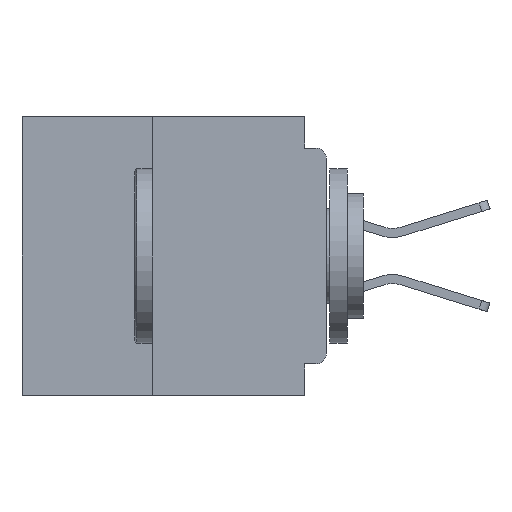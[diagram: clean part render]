
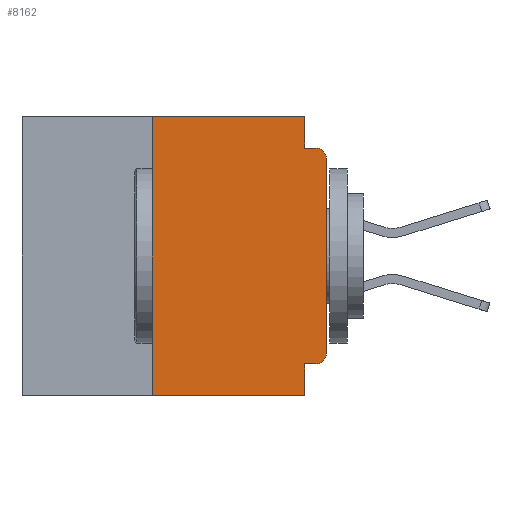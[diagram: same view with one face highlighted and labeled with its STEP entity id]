
A CAD part, left-side view. The second image highlights one B-rep face of the part: STEP entity #8162.
In plain terms, the highlighted planar face has unit normal (-1, 0, 0).
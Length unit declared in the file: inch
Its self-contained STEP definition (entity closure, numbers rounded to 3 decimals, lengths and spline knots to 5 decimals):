
#472 = DIRECTION ( 'NONE',  ( 0., 0., -1. ) ) ;
#591 = VECTOR ( 'NONE', #36430, 39.37008 ) ;
#720 = VECTOR ( 'NONE', #472, 39.37008 ) ;
#1626 = CARTESIAN_POINT ( 'NONE',  ( 0., 0., -0.045 ) ) ;
#1841 = VERTEX_POINT ( 'NONE', #35062 ) ;
#2257 = LINE ( 'NONE', #1626, #17665 ) ;
#2867 = VERTEX_POINT ( 'NONE', #30330 ) ;
#3822 = DIRECTION ( 'NONE',  ( 0., 0., -1. ) ) ;
#4302 = ORIENTED_EDGE ( 'NONE', *, *, #34693, .T. ) ;
#4424 = EDGE_CURVE ( 'NONE', #17316, #37207, #24760, .T. ) ;
#4809 = EDGE_LOOP ( 'NONE', ( #5668, #30930, #11366, #27231, #41354, #8035, #8741, #14211, #24919, #4302 ) ) ;
#5165 = AXIS2_PLACEMENT_3D ( 'NONE', #16802, #23419, #3822 ) ;
#5299 = CARTESIAN_POINT ( 'NONE',  ( 0., 0., -0.34 ) ) ;
#5668 = ORIENTED_EDGE ( 'NONE', *, *, #7527, .T. ) ;
#6003 = CARTESIAN_POINT ( 'NONE',  ( 0., 0.015, -0.045 ) ) ;
#6198 = CARTESIAN_POINT ( 'NONE',  ( 0., 0.437, -0.4 ) ) ;
#6359 = EDGE_CURVE ( 'NONE', #32791, #16453, #21707, .T. ) ;
#6423 = VECTOR ( 'NONE', #14970, 39.37008 ) ;
#7133 = CARTESIAN_POINT ( 'NONE',  ( 0., 0.031, -0.4 ) ) ;
#7527 = EDGE_CURVE ( 'NONE', #12212, #1841, #34368, .T. ) ;
#7808 = CIRCLE ( 'NONE', #42087, 0.015 ) ;
#8035 = ORIENTED_EDGE ( 'NONE', *, *, #19155, .F. ) ;
#8162 = ADVANCED_FACE ( 'NONE', ( #29196 ), #16932, .F. ) ;
#8741 = ORIENTED_EDGE ( 'NONE', *, *, #30692, .T. ) ;
#9673 = VECTOR ( 'NONE', #9690, 39.37008 ) ;
#9690 = DIRECTION ( 'NONE',  ( 0., -1., 0. ) ) ;
#10240 = CARTESIAN_POINT ( 'NONE',  ( 0., 0.015, -0.355 ) ) ;
#11366 = ORIENTED_EDGE ( 'NONE', *, *, #16310, .F. ) ;
#11463 = EDGE_CURVE ( 'NONE', #16453, #18446, #32494, .T. ) ;
#12212 = VERTEX_POINT ( 'NONE', #5299 ) ;
#13723 = CARTESIAN_POINT ( 'NONE',  ( 0., 0., 0. ) ) ;
#14105 = CARTESIAN_POINT ( 'NONE',  ( 0., 0.437, 0. ) ) ;
#14211 = ORIENTED_EDGE ( 'NONE', *, *, #16106, .F. ) ;
#14970 = DIRECTION ( 'NONE',  ( 0., 0., -1. ) ) ;
#15608 = CARTESIAN_POINT ( 'NONE',  ( 0., 0.031, 0. ) ) ;
#16106 = EDGE_CURVE ( 'NONE', #37207, #2867, #34491, .T. ) ;
#16310 = EDGE_CURVE ( 'NONE', #18446, #29494, #2257, .T. ) ;
#16453 = VERTEX_POINT ( 'NONE', #15608 ) ;
#16802 = CARTESIAN_POINT ( 'NONE',  ( 0., 0.437, 0. ) ) ;
#16932 = PLANE ( 'NONE',  #5165 ) ;
#16974 = CARTESIAN_POINT ( 'NONE',  ( 0., 0.015, -0.06 ) ) ;
#17092 = DIRECTION ( 'NONE',  ( -1., 0., 0. ) ) ;
#17316 = VERTEX_POINT ( 'NONE', #10240 ) ;
#17620 = CARTESIAN_POINT ( 'NONE',  ( 0., 0.031, -0.045 ) ) ;
#17665 = VECTOR ( 'NONE', #17990, 39.37008 ) ;
#17990 = DIRECTION ( 'NONE',  ( 0., -1., 0. ) ) ;
#18341 = LINE ( 'NONE', #6198, #9673 ) ;
#18446 = VERTEX_POINT ( 'NONE', #17620 ) ;
#19155 = EDGE_CURVE ( 'NONE', #29608, #32791, #33899, .T. ) ;
#20200 = DIRECTION ( 'NONE',  ( 0., 0., -1. ) ) ;
#20693 = VECTOR ( 'NONE', #33583, 39.37008 ) ;
#20838 = CIRCLE ( 'NONE', #38742, 0.015 ) ;
#21707 = LINE ( 'NONE', #14105, #20693 ) ;
#22819 = CARTESIAN_POINT ( 'NONE',  ( 0., 0.25, -0.4 ) ) ;
#23005 = CARTESIAN_POINT ( 'NONE',  ( 0., 0.25, 0. ) ) ;
#23419 = DIRECTION ( 'NONE',  ( 1., 0., 0. ) ) ;
#24572 = CARTESIAN_POINT ( 'NONE',  ( 0., 0.031, 0. ) ) ;
#24760 = LINE ( 'NONE', #38075, #32406 ) ;
#24919 = ORIENTED_EDGE ( 'NONE', *, *, #4424, .F. ) ;
#25226 = VECTOR ( 'NONE', #34357, 39.37008 ) ;
#25429 = CARTESIAN_POINT ( 'NONE',  ( 0., 0.031, -0.355 ) ) ;
#27231 = ORIENTED_EDGE ( 'NONE', *, *, #11463, .F. ) ;
#29196 = FACE_OUTER_BOUND ( 'NONE', #4809, .T. ) ;
#29494 = VERTEX_POINT ( 'NONE', #6003 ) ;
#29608 = VERTEX_POINT ( 'NONE', #22819 ) ;
#30330 = CARTESIAN_POINT ( 'NONE',  ( 0., 0.031, -0.4 ) ) ;
#30692 = EDGE_CURVE ( 'NONE', #29608, #2867, #18341, .T. ) ;
#30930 = ORIENTED_EDGE ( 'NONE', *, *, #40785, .T. ) ;
#32406 = VECTOR ( 'NONE', #38083, 39.37008 ) ;
#32494 = LINE ( 'NONE', #24572, #6423 ) ;
#32791 = VERTEX_POINT ( 'NONE', #23005 ) ;
#33583 = DIRECTION ( 'NONE',  ( 0., -1., 0. ) ) ;
#33899 = LINE ( 'NONE', #40755, #25226 ) ;
#34357 = DIRECTION ( 'NONE',  ( 0., 0., 1. ) ) ;
#34368 = LINE ( 'NONE', #13723, #591 ) ;
#34491 = LINE ( 'NONE', #7133, #720 ) ;
#34693 = EDGE_CURVE ( 'NONE', #17316, #12212, #7808, .T. ) ;
#35062 = CARTESIAN_POINT ( 'NONE',  ( 0., 0., -0.06 ) ) ;
#36430 = DIRECTION ( 'NONE',  ( 0., 0., 1. ) ) ;
#36547 = CARTESIAN_POINT ( 'NONE',  ( 0., 0.015, -0.34 ) ) ;
#37207 = VERTEX_POINT ( 'NONE', #25429 ) ;
#38075 = CARTESIAN_POINT ( 'NONE',  ( 0., 0., -0.355 ) ) ;
#38083 = DIRECTION ( 'NONE',  ( 0., 1., 0. ) ) ;
#38742 = AXIS2_PLACEMENT_3D ( 'NONE', #16974, #39697, #20200 ) ;
#39697 = DIRECTION ( 'NONE',  ( -1., 0., 0. ) ) ;
#39822 = DIRECTION ( 'NONE',  ( 0., 0., -1. ) ) ;
#40755 = CARTESIAN_POINT ( 'NONE',  ( 0., 0.25, -0.4 ) ) ;
#40785 = EDGE_CURVE ( 'NONE', #1841, #29494, #20838, .T. ) ;
#41354 = ORIENTED_EDGE ( 'NONE', *, *, #6359, .F. ) ;
#42087 = AXIS2_PLACEMENT_3D ( 'NONE', #36547, #17092, #39822 ) ;
